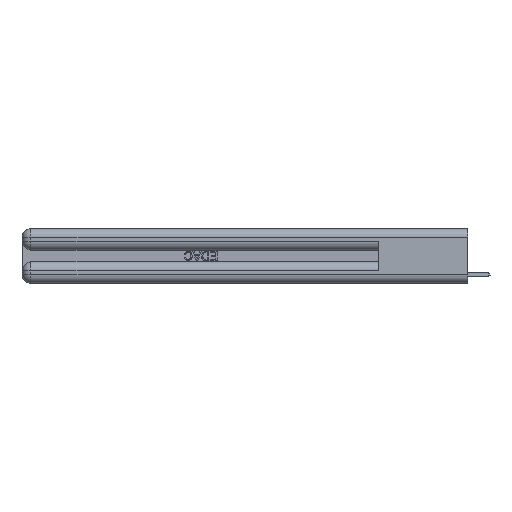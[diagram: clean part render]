
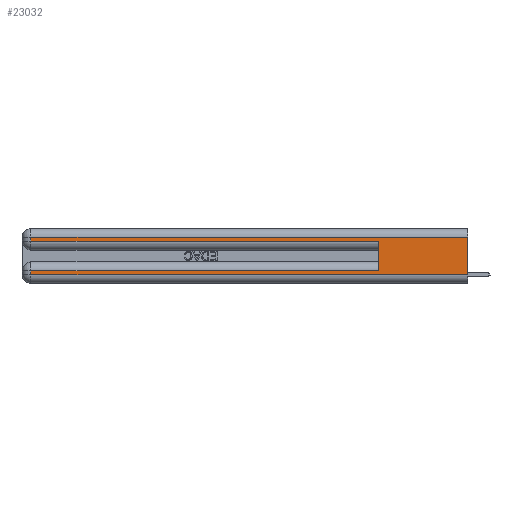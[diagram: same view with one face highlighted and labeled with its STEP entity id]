
A CAD part, left-side view. The second image highlights one B-rep face of the part: STEP entity #23032.
In plain terms, the highlighted planar face has unit normal (-1, 0, 0).
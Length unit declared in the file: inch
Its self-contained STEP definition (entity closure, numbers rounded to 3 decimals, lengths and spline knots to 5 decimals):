
#1448 = VECTOR ( 'NONE', #11336, 39.37008 ) ;
#1449 = CARTESIAN_POINT ( 'NONE',  ( 0., 0., 0.085 ) ) ;
#2286 = CARTESIAN_POINT ( 'NONE',  ( 0., 2.94, 0.31 ) ) ;
#2326 = CARTESIAN_POINT ( 'NONE',  ( 0., 2.94, 0.37 ) ) ;
#2342 = EDGE_CURVE ( 'NONE', #20713, #23666, #2771, .T. ) ;
#2359 = DIRECTION ( 'NONE',  ( 0., 0., 1. ) ) ;
#2656 = LINE ( 'NONE', #13286, #10188 ) ;
#2680 = EDGE_LOOP ( 'NONE', ( #24610, #27389, #24858, #9662, #16914, #4803, #7659, #3654 ) ) ;
#2771 = LINE ( 'NONE', #27836, #7170 ) ;
#2796 = EDGE_CURVE ( 'NONE', #9181, #5410, #13653, .T. ) ;
#2944 = LINE ( 'NONE', #20910, #26313 ) ;
#3654 = ORIENTED_EDGE ( 'NONE', *, *, #2342, .T. ) ;
#3685 = DIRECTION ( 'NONE',  ( 0., 1., 0. ) ) ;
#4211 = VECTOR ( 'NONE', #17766, 39.37008 ) ;
#4771 = CARTESIAN_POINT ( 'NONE',  ( 0., 0.6, 0.085 ) ) ;
#4803 = ORIENTED_EDGE ( 'NONE', *, *, #8149, .T. ) ;
#5328 = DIRECTION ( 'NONE',  ( 0., 0., -1. ) ) ;
#5410 = VERTEX_POINT ( 'NONE', #9206 ) ;
#5955 = LINE ( 'NONE', #24060, #27217 ) ;
#6686 = VECTOR ( 'NONE', #20393, 39.37008 ) ;
#6692 = LINE ( 'NONE', #24204, #4211 ) ;
#7170 = VECTOR ( 'NONE', #25354, 39.37008 ) ;
#7374 = CARTESIAN_POINT ( 'NONE',  ( 0., 2.94, 0.085 ) ) ;
#7659 = ORIENTED_EDGE ( 'NONE', *, *, #10130, .T. ) ;
#8149 = EDGE_CURVE ( 'NONE', #29174, #28047, #26083, .T. ) ;
#8709 = LINE ( 'NONE', #2326, #1448 ) ;
#9181 = VERTEX_POINT ( 'NONE', #20981 ) ;
#9206 = CARTESIAN_POINT ( 'NONE',  ( 0., 0.6, 0.285 ) ) ;
#9662 = ORIENTED_EDGE ( 'NONE', *, *, #2796, .T. ) ;
#10130 = EDGE_CURVE ( 'NONE', #28047, #20713, #6692, .T. ) ;
#10188 = VECTOR ( 'NONE', #2359, 39.37008 ) ;
#11336 = DIRECTION ( 'NONE',  ( 0., 0., -1. ) ) ;
#11806 = EDGE_CURVE ( 'NONE', #14430, #9181, #8709, .T. ) ;
#12159 = FACE_OUTER_BOUND ( 'NONE', #2680, .T. ) ;
#13286 = CARTESIAN_POINT ( 'NONE',  ( 0., 0.6, 0.145 ) ) ;
#13653 = LINE ( 'NONE', #24405, #6686 ) ;
#13999 = EDGE_CURVE ( 'NONE', #20491, #14430, #5955, .T. ) ;
#14430 = VERTEX_POINT ( 'NONE', #2286 ) ;
#15221 = CARTESIAN_POINT ( 'NONE',  ( 0., 2.94, 0.06 ) ) ;
#15543 = EDGE_CURVE ( 'NONE', #29174, #5410, #2656, .T. ) ;
#15605 = EDGE_CURVE ( 'NONE', #20491, #23666, #2944, .T. ) ;
#16773 = CARTESIAN_POINT ( 'NONE',  ( 0., 0., 0.37 ) ) ;
#16914 = ORIENTED_EDGE ( 'NONE', *, *, #15543, .F. ) ;
#17766 = DIRECTION ( 'NONE',  ( 0., 0., -1. ) ) ;
#17946 = DIRECTION ( 'NONE',  ( 0., 0., -1. ) ) ;
#17998 = CARTESIAN_POINT ( 'NONE',  ( 0., 0., 0.06 ) ) ;
#18202 = CARTESIAN_POINT ( 'NONE',  ( 0., 0., 0.31 ) ) ;
#19042 = PLANE ( 'NONE',  #21521 ) ;
#19900 = DIRECTION ( 'NONE',  ( 1., 0., 0. ) ) ;
#20393 = DIRECTION ( 'NONE',  ( 0., -1., 0. ) ) ;
#20491 = VERTEX_POINT ( 'NONE', #18202 ) ;
#20713 = VERTEX_POINT ( 'NONE', #15221 ) ;
#20910 = CARTESIAN_POINT ( 'NONE',  ( 0., 0., 0.37 ) ) ;
#20981 = CARTESIAN_POINT ( 'NONE',  ( 0., 2.94, 0.285 ) ) ;
#21474 = DIRECTION ( 'NONE',  ( 0., 1., 0. ) ) ;
#21521 = AXIS2_PLACEMENT_3D ( 'NONE', #16773, #19900, #17946 ) ;
#23032 = ADVANCED_FACE ( 'NONE', ( #12159 ), #19042, .F. ) ;
#23666 = VERTEX_POINT ( 'NONE', #17998 ) ;
#24060 = CARTESIAN_POINT ( 'NONE',  ( 0., 0., 0.31 ) ) ;
#24204 = CARTESIAN_POINT ( 'NONE',  ( 0., 2.94, 0.37 ) ) ;
#24405 = CARTESIAN_POINT ( 'NONE',  ( 0., 0., 0.285 ) ) ;
#24610 = ORIENTED_EDGE ( 'NONE', *, *, #15605, .F. ) ;
#24858 = ORIENTED_EDGE ( 'NONE', *, *, #11806, .T. ) ;
#25354 = DIRECTION ( 'NONE',  ( 0., -1., 0. ) ) ;
#26083 = LINE ( 'NONE', #1449, #26363 ) ;
#26313 = VECTOR ( 'NONE', #5328, 39.37008 ) ;
#26363 = VECTOR ( 'NONE', #21474, 39.37008 ) ;
#27217 = VECTOR ( 'NONE', #3685, 39.37008 ) ;
#27389 = ORIENTED_EDGE ( 'NONE', *, *, #13999, .T. ) ;
#27836 = CARTESIAN_POINT ( 'NONE',  ( 0., 0., 0.06 ) ) ;
#28047 = VERTEX_POINT ( 'NONE', #7374 ) ;
#29174 = VERTEX_POINT ( 'NONE', #4771 ) ;
